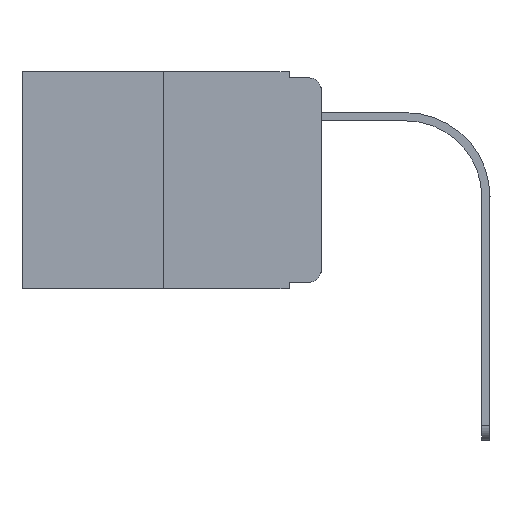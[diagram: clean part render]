
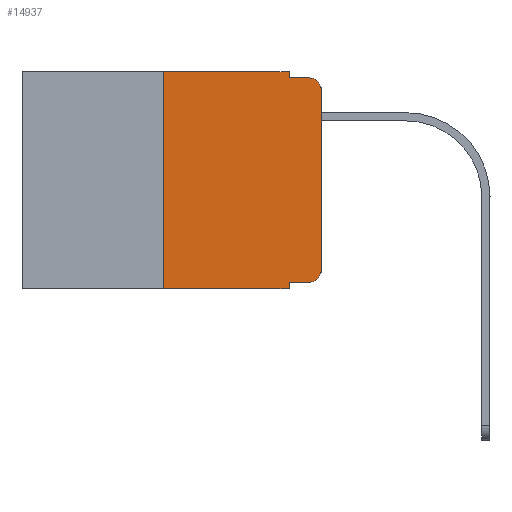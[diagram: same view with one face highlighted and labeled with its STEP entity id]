
A CAD part, left-side view. The second image highlights one B-rep face of the part: STEP entity #14937.
In plain terms, the highlighted planar face has unit normal (-1, 0, 0).
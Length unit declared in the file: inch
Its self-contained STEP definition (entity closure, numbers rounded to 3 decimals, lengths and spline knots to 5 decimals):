
#131 = ORIENTED_EDGE ( 'NONE', *, *, #5168, .T. ) ;
#1213 = LINE ( 'NONE', #12109, #4386 ) ;
#1347 = ORIENTED_EDGE ( 'NONE', *, *, #14332, .F. ) ;
#1586 = EDGE_CURVE ( 'NONE', #8345, #16354, #2132, .T. ) ;
#1784 = EDGE_CURVE ( 'NONE', #5883, #18186, #2491, .T. ) ;
#2117 = CARTESIAN_POINT ( 'NONE',  ( 0., 0., -0.313 ) ) ;
#2132 = CIRCLE ( 'NONE', #13380, 0.02 ) ;
#2491 = CIRCLE ( 'NONE', #12019, 0.02 ) ;
#2993 = DIRECTION ( 'NONE',  ( 0., 0., -1. ) ) ;
#3014 = EDGE_CURVE ( 'NONE', #9110, #7022, #19159, .T. ) ;
#3392 = LINE ( 'NONE', #19399, #7489 ) ;
#3976 = ORIENTED_EDGE ( 'NONE', *, *, #12224, .F. ) ;
#3980 = CARTESIAN_POINT ( 'NONE',  ( 0., 0.051, -0.01 ) ) ;
#4321 = DIRECTION ( 'NONE',  ( 0., 0., -1. ) ) ;
#4386 = VECTOR ( 'NONE', #14122, 39.37008 ) ;
#4772 = DIRECTION ( 'NONE',  ( 0., -1., 0. ) ) ;
#4921 = ORIENTED_EDGE ( 'NONE', *, *, #16539, .F. ) ;
#5168 = EDGE_CURVE ( 'NONE', #18186, #8345, #1213, .T. ) ;
#5725 = LINE ( 'NONE', #11810, #6622 ) ;
#5727 = EDGE_CURVE ( 'NONE', #19380, #18389, #7166, .T. ) ;
#5883 = VERTEX_POINT ( 'NONE', #16766 ) ;
#6197 = ORIENTED_EDGE ( 'NONE', *, *, #3014, .F. ) ;
#6406 = DIRECTION ( 'NONE',  ( 1., 0., 0. ) ) ;
#6622 = VECTOR ( 'NONE', #15554, 39.37008 ) ;
#6839 = LINE ( 'NONE', #14964, #17507 ) ;
#6907 = CARTESIAN_POINT ( 'NONE',  ( 0., 0.051, -0.343 ) ) ;
#7022 = VERTEX_POINT ( 'NONE', #3980 ) ;
#7150 = DIRECTION ( 'NONE',  ( 0., 0., -1. ) ) ;
#7166 = LINE ( 'NONE', #20427, #16019 ) ;
#7489 = VECTOR ( 'NONE', #4772, 39.37008 ) ;
#7586 = DIRECTION ( 'NONE',  ( 0., 0., 1. ) ) ;
#7808 = LINE ( 'NONE', #11124, #10780 ) ;
#8267 = CARTESIAN_POINT ( 'NONE',  ( 0., 0.051, -0.333 ) ) ;
#8345 = VERTEX_POINT ( 'NONE', #10619 ) ;
#8446 = ORIENTED_EDGE ( 'NONE', *, *, #1586, .T. ) ;
#8755 = CARTESIAN_POINT ( 'NONE',  ( 0., 0.051, 0. ) ) ;
#8777 = DIRECTION ( 'NONE',  ( -1., 0., 0. ) ) ;
#8849 = CARTESIAN_POINT ( 'NONE',  ( 0., 0.02, -0.01 ) ) ;
#9110 = VERTEX_POINT ( 'NONE', #8755 ) ;
#9113 = CARTESIAN_POINT ( 'NONE',  ( 0., 0.02, -0.03 ) ) ;
#9150 = ORIENTED_EDGE ( 'NONE', *, *, #9554, .T. ) ;
#9301 = EDGE_LOOP ( 'NONE', ( #131, #8446, #1347, #6197, #4921, #11516, #14844, #3976, #9150, #18541 ) ) ;
#9341 = CARTESIAN_POINT ( 'NONE',  ( 0., 0.051, 0. ) ) ;
#9418 = DIRECTION ( 'NONE',  ( -1., 0., 0. ) ) ;
#9554 = EDGE_CURVE ( 'NONE', #14055, #5883, #5725, .T. ) ;
#9688 = VECTOR ( 'NONE', #4321, 39.37008 ) ;
#10619 = CARTESIAN_POINT ( 'NONE',  ( 0., 0., -0.03 ) ) ;
#10723 = VERTEX_POINT ( 'NONE', #6907 ) ;
#10780 = VECTOR ( 'NONE', #14210, 39.37008 ) ;
#11124 = CARTESIAN_POINT ( 'NONE',  ( 0., 0.051, -0.01 ) ) ;
#11137 = DIRECTION ( 'NONE',  ( 0., -1., 0. ) ) ;
#11416 = CARTESIAN_POINT ( 'NONE',  ( 0., 0.25, -0.343 ) ) ;
#11516 = ORIENTED_EDGE ( 'NONE', *, *, #5727, .F. ) ;
#11810 = CARTESIAN_POINT ( 'NONE',  ( 0., 0.051, -0.333 ) ) ;
#12019 = AXIS2_PLACEMENT_3D ( 'NONE', #14426, #8777, #18286 ) ;
#12109 = CARTESIAN_POINT ( 'NONE',  ( 0., 0., 0. ) ) ;
#12224 = EDGE_CURVE ( 'NONE', #14055, #10723, #6839, .T. ) ;
#13054 = LINE ( 'NONE', #14558, #13244 ) ;
#13244 = VECTOR ( 'NONE', #11137, 39.37008 ) ;
#13380 = AXIS2_PLACEMENT_3D ( 'NONE', #9113, #9418, #13910 ) ;
#13408 = FACE_OUTER_BOUND ( 'NONE', #9301, .T. ) ;
#13910 = DIRECTION ( 'NONE',  ( 0., 0., -1. ) ) ;
#14055 = VERTEX_POINT ( 'NONE', #8267 ) ;
#14122 = DIRECTION ( 'NONE',  ( 0., 0., 1. ) ) ;
#14210 = DIRECTION ( 'NONE',  ( 0., -1., 0. ) ) ;
#14332 = EDGE_CURVE ( 'NONE', #7022, #16354, #7808, .T. ) ;
#14426 = CARTESIAN_POINT ( 'NONE',  ( 0., 0.02, -0.313 ) ) ;
#14513 = CARTESIAN_POINT ( 'NONE',  ( 0., 0.473, 0. ) ) ;
#14558 = CARTESIAN_POINT ( 'NONE',  ( 0., 0.473, -0.343 ) ) ;
#14844 = ORIENTED_EDGE ( 'NONE', *, *, #17228, .T. ) ;
#14937 = ADVANCED_FACE ( 'NONE', ( #13408 ), #17837, .F. ) ;
#14964 = CARTESIAN_POINT ( 'NONE',  ( 0., 0.051, 0. ) ) ;
#15554 = DIRECTION ( 'NONE',  ( 0., -1., 0. ) ) ;
#15568 = AXIS2_PLACEMENT_3D ( 'NONE', #14513, #6406, #2993 ) ;
#16019 = VECTOR ( 'NONE', #7586, 39.37008 ) ;
#16354 = VERTEX_POINT ( 'NONE', #8849 ) ;
#16539 = EDGE_CURVE ( 'NONE', #18389, #9110, #3392, .T. ) ;
#16766 = CARTESIAN_POINT ( 'NONE',  ( 0., 0.02, -0.333 ) ) ;
#17228 = EDGE_CURVE ( 'NONE', #19380, #10723, #13054, .T. ) ;
#17507 = VECTOR ( 'NONE', #7150, 39.37008 ) ;
#17837 = PLANE ( 'NONE',  #15568 ) ;
#18186 = VERTEX_POINT ( 'NONE', #2117 ) ;
#18286 = DIRECTION ( 'NONE',  ( 0., 0., -1. ) ) ;
#18389 = VERTEX_POINT ( 'NONE', #18886 ) ;
#18541 = ORIENTED_EDGE ( 'NONE', *, *, #1784, .T. ) ;
#18886 = CARTESIAN_POINT ( 'NONE',  ( 0., 0.25, 0. ) ) ;
#19159 = LINE ( 'NONE', #9341, #9688 ) ;
#19380 = VERTEX_POINT ( 'NONE', #11416 ) ;
#19399 = CARTESIAN_POINT ( 'NONE',  ( 0., 0.473, 0. ) ) ;
#20427 = CARTESIAN_POINT ( 'NONE',  ( 0., 0.25, 0. ) ) ;
